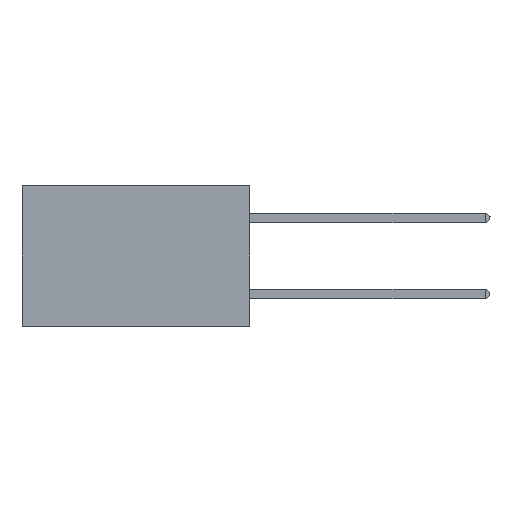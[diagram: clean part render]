
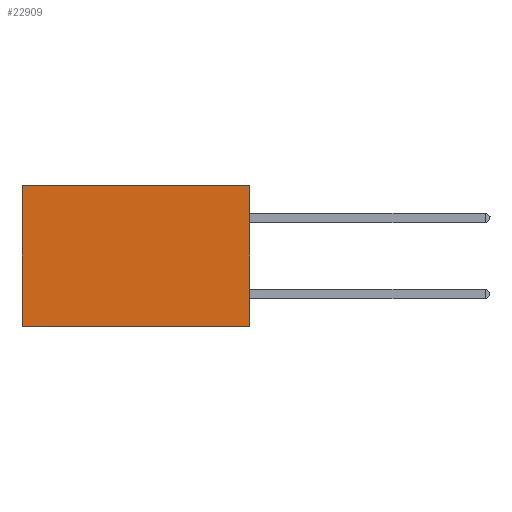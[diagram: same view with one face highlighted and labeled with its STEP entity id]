
A CAD part, left-side view. The second image highlights one B-rep face of the part: STEP entity #22909.
In plain terms, the highlighted planar face has unit normal (-1, 0, 0).
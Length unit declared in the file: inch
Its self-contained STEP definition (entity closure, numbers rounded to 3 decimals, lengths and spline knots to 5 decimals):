
#783 = DIRECTION ( 'NONE',  ( 0., 0., -1. ) ) ;
#1170 = ORIENTED_EDGE ( 'NONE', *, *, #12138, .F. ) ;
#1691 = DIRECTION ( 'NONE',  ( 1., 0., 0. ) ) ;
#2078 = FACE_OUTER_BOUND ( 'NONE', #18997, .T. ) ;
#2270 = VERTEX_POINT ( 'NONE', #2950 ) ;
#2950 = CARTESIAN_POINT ( 'NONE',  ( 0.2875, 0., 0. ) ) ;
#3698 = PLANE ( 'NONE',  #5809 ) ;
#3916 = LINE ( 'NONE', #23905, #11743 ) ;
#5781 = CARTESIAN_POINT ( 'NONE',  ( 0.2875, 0.6, -0.37 ) ) ;
#5809 = AXIS2_PLACEMENT_3D ( 'NONE', #20437, #1691, #16032 ) ;
#7109 = LINE ( 'NONE', #19952, #7756 ) ;
#7627 = CARTESIAN_POINT ( 'NONE',  ( 0.2875, 0.6, 0. ) ) ;
#7756 = VECTOR ( 'NONE', #26248, 39.37008 ) ;
#8775 = VECTOR ( 'NONE', #26951, 39.37008 ) ;
#11743 = VECTOR ( 'NONE', #783, 39.37008 ) ;
#11910 = EDGE_CURVE ( 'NONE', #2270, #17227, #7109, .T. ) ;
#12138 = EDGE_CURVE ( 'NONE', #19985, #15093, #17588, .T. ) ;
#12481 = CARTESIAN_POINT ( 'NONE',  ( 0.2875, 0., 0. ) ) ;
#13422 = ORIENTED_EDGE ( 'NONE', *, *, #16750, .T. ) ;
#13665 = LINE ( 'NONE', #12481, #8775 ) ;
#14725 = ORIENTED_EDGE ( 'NONE', *, *, #17432, .F. ) ;
#15093 = VERTEX_POINT ( 'NONE', #5781 ) ;
#16032 = DIRECTION ( 'NONE',  ( 0., 0., -1. ) ) ;
#16750 = EDGE_CURVE ( 'NONE', #17227, #15093, #3916, .T. ) ;
#16895 = CARTESIAN_POINT ( 'NONE',  ( 0.2875, 0., -0.37 ) ) ;
#17227 = VERTEX_POINT ( 'NONE', #7627 ) ;
#17432 = EDGE_CURVE ( 'NONE', #2270, #19985, #13665, .T. ) ;
#17588 = LINE ( 'NONE', #23450, #21869 ) ;
#18997 = EDGE_LOOP ( 'NONE', ( #13422, #1170, #14725, #24250 ) ) ;
#19952 = CARTESIAN_POINT ( 'NONE',  ( 0.2875, 0., 0. ) ) ;
#19985 = VERTEX_POINT ( 'NONE', #16895 ) ;
#20437 = CARTESIAN_POINT ( 'NONE',  ( 0.2875, 0., 0. ) ) ;
#21869 = VECTOR ( 'NONE', #22967, 39.37008 ) ;
#22909 = ADVANCED_FACE ( 'NONE', ( #2078 ), #3698, .F. ) ;
#22967 = DIRECTION ( 'NONE',  ( 0., 1., 0. ) ) ;
#23450 = CARTESIAN_POINT ( 'NONE',  ( 0.2875, 0., -0.37 ) ) ;
#23905 = CARTESIAN_POINT ( 'NONE',  ( 0.2875, 0.6, 0. ) ) ;
#24250 = ORIENTED_EDGE ( 'NONE', *, *, #11910, .T. ) ;
#26248 = DIRECTION ( 'NONE',  ( 0., 1., 0. ) ) ;
#26951 = DIRECTION ( 'NONE',  ( 0., 0., -1. ) ) ;
